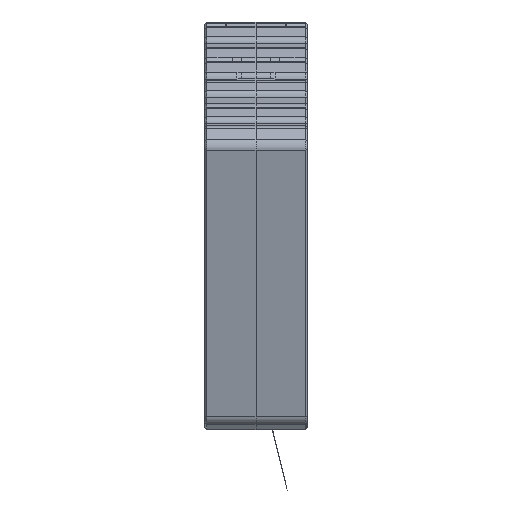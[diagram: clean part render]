
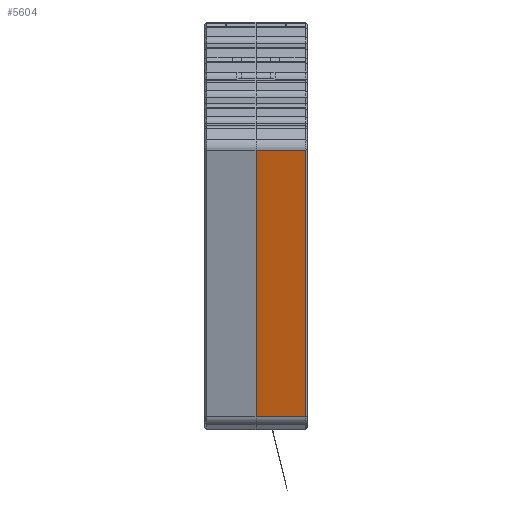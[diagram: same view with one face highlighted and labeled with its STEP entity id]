
A CAD part, front view. The second image highlights one B-rep face of the part: STEP entity #5604.
In plain terms, the highlighted planar face has unit normal (0, -0.97, -0.241).
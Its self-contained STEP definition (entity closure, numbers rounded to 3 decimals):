
#5604 = ADVANCED_FACE ( 'NONE', ( #128250 ), #116419, .T. ) ;
#6519 = CARTESIAN_POINT ( 'NONE',  ( 12.252, -160.79, 10.379 ) ) ;
#8856 = DIRECTION ( 'NONE',  ( 1., 0., 0. ) ) ;
#9190 = DIRECTION ( 'NONE',  ( -1., 0., 0. ) ) ;
#12251 = EDGE_CURVE ( 'NONE', #82685, #140241, #121965, .T. ) ;
#20328 = EDGE_CURVE ( 'NONE', #109894, #24159, #54411, .T. ) ;
#22575 = VECTOR ( 'NONE', #124125, 1000. ) ;
#24159 = VERTEX_POINT ( 'NONE', #110813 ) ;
#24436 = EDGE_CURVE ( 'NONE', #140241, #24159, #144589, .T. ) ;
#25574 = ORIENTED_EDGE ( 'NONE', *, *, #24436, .F. ) ;
#38193 = CARTESIAN_POINT ( 'NONE',  ( 0., -160.79, 10.379 ) ) ;
#48795 = EDGE_LOOP ( 'NONE', ( #120305, #97969, #25574, #94669 ) ) ;
#53586 = CARTESIAN_POINT ( 'NONE',  ( 110.954, -144.332, -55.775 ) ) ;
#54411 = LINE ( 'NONE', #98029, #68790 ) ;
#60773 = AXIS2_PLACEMENT_3D ( 'NONE', #106041, #83848, #72724 ) ;
#68790 = VECTOR ( 'NONE', #98756, 1000. ) ;
#72724 = DIRECTION ( 'NONE',  ( 0., 0.241, -0.97 ) ) ;
#72841 = EDGE_CURVE ( 'NONE', #109894, #82685, #120600, .T. ) ;
#82685 = VERTEX_POINT ( 'NONE', #6519 ) ;
#83848 = DIRECTION ( 'NONE',  ( 0., -0.97, -0.241 ) ) ;
#88731 = CARTESIAN_POINT ( 'NONE',  ( 110.954, -160.79, 10.379 ) ) ;
#94669 = ORIENTED_EDGE ( 'NONE', *, *, #12251, .F. ) ;
#97969 = ORIENTED_EDGE ( 'NONE', *, *, #20328, .T. ) ;
#98029 = CARTESIAN_POINT ( 'NONE',  ( 0., -144.69, -54.333 ) ) ;
#98756 = DIRECTION ( 'NONE',  ( 0., 0.241, -0.97 ) ) ;
#101191 = CARTESIAN_POINT ( 'NONE',  ( 12.252, -144.69, -54.333 ) ) ;
#106041 = CARTESIAN_POINT ( 'NONE',  ( 110.954, -144.69, -54.333 ) ) ;
#109894 = VERTEX_POINT ( 'NONE', #38193 ) ;
#110813 = CARTESIAN_POINT ( 'NONE',  ( 0., -144.332, -55.775 ) ) ;
#116419 = PLANE ( 'NONE',  #60773 ) ;
#118758 = CARTESIAN_POINT ( 'NONE',  ( 12.252, -144.332, -55.775 ) ) ;
#120305 = ORIENTED_EDGE ( 'NONE', *, *, #72841, .F. ) ;
#120600 = LINE ( 'NONE', #88731, #123728 ) ;
#121965 = LINE ( 'NONE', #101191, #22575 ) ;
#123728 = VECTOR ( 'NONE', #8856, 1000. ) ;
#124125 = DIRECTION ( 'NONE',  ( 0., 0.241, -0.97 ) ) ;
#128250 = FACE_OUTER_BOUND ( 'NONE', #48795, .T. ) ;
#134429 = VECTOR ( 'NONE', #9190, 1000. ) ;
#140241 = VERTEX_POINT ( 'NONE', #118758 ) ;
#144589 = LINE ( 'NONE', #53586, #134429 ) ;
